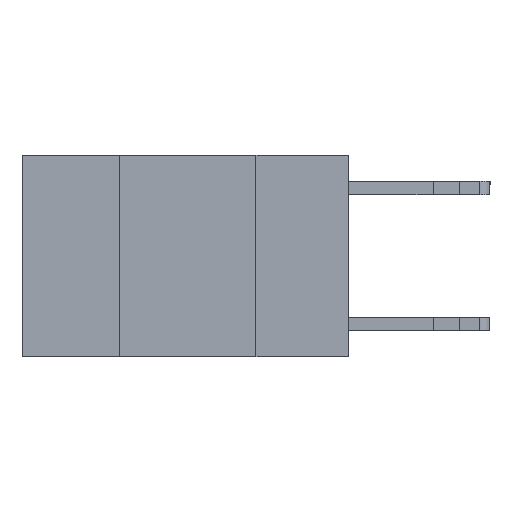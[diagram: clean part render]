
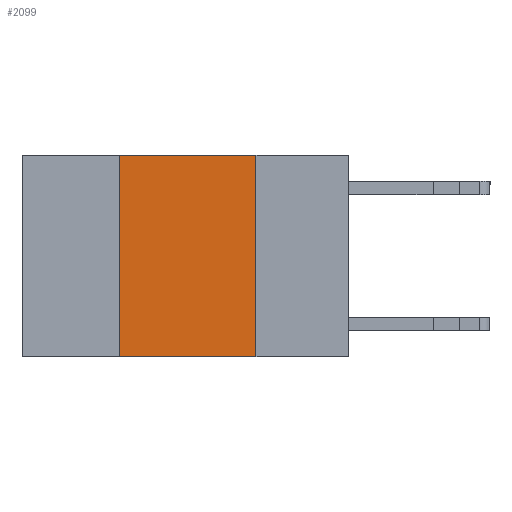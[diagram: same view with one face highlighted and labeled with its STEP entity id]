
A CAD part, left-side view. The second image highlights one B-rep face of the part: STEP entity #2099.
In plain terms, the highlighted planar face has unit normal (-1, 0, 0).
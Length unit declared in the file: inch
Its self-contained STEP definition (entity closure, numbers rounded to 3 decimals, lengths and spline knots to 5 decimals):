
#882 = CARTESIAN_POINT ( 'NONE',  ( 0., 0.17, -0.37 ) ) ;
#1571 = DIRECTION ( 'NONE',  ( 0., 0., -1. ) ) ;
#1668 = AXIS2_PLACEMENT_3D ( 'NONE', #8676, #10941, #1571 ) ;
#1819 = DIRECTION ( 'NONE',  ( 0., -1., 0. ) ) ;
#2099 = ADVANCED_FACE ( 'NONE', ( #13008 ), #7789, .F. ) ;
#2746 = ORIENTED_EDGE ( 'NONE', *, *, #3608, .F. ) ;
#3571 = VERTEX_POINT ( 'NONE', #882 ) ;
#3608 = EDGE_CURVE ( 'NONE', #10512, #7914, #11284, .T. ) ;
#3910 = CARTESIAN_POINT ( 'NONE',  ( 0., 0.17, 0. ) ) ;
#3930 = VECTOR ( 'NONE', #1819, 39.37008 ) ;
#4198 = EDGE_LOOP ( 'NONE', ( #11548, #12940, #2746, #7398 ) ) ;
#4563 = CARTESIAN_POINT ( 'NONE',  ( 0., 0.42, -0.37 ) ) ;
#4791 = VECTOR ( 'NONE', #10331, 39.37008 ) ;
#5809 = LINE ( 'NONE', #12005, #11822 ) ;
#6104 = EDGE_CURVE ( 'NONE', #7914, #10002, #5809, .T. ) ;
#6196 = EDGE_CURVE ( 'NONE', #10002, #3571, #8201, .T. ) ;
#7398 = ORIENTED_EDGE ( 'NONE', *, *, #12355, .T. ) ;
#7789 = PLANE ( 'NONE',  #1668 ) ;
#7914 = VERTEX_POINT ( 'NONE', #8962 ) ;
#8201 = LINE ( 'NONE', #3910, #4791 ) ;
#8676 = CARTESIAN_POINT ( 'NONE',  ( 0., 0.6, 0. ) ) ;
#8962 = CARTESIAN_POINT ( 'NONE',  ( 0., 0.42, 0. ) ) ;
#9032 = DIRECTION ( 'NONE',  ( 0., 0., 1. ) ) ;
#9234 = CARTESIAN_POINT ( 'NONE',  ( 0., 0.42, 0. ) ) ;
#9805 = DIRECTION ( 'NONE',  ( 0., -1., 0. ) ) ;
#10002 = VERTEX_POINT ( 'NONE', #12955 ) ;
#10331 = DIRECTION ( 'NONE',  ( 0., 0., -1. ) ) ;
#10512 = VERTEX_POINT ( 'NONE', #4563 ) ;
#10941 = DIRECTION ( 'NONE',  ( 1., 0., 0. ) ) ;
#11198 = CARTESIAN_POINT ( 'NONE',  ( 0., 0.6, -0.37 ) ) ;
#11284 = LINE ( 'NONE', #9234, #11762 ) ;
#11548 = ORIENTED_EDGE ( 'NONE', *, *, #6196, .F. ) ;
#11762 = VECTOR ( 'NONE', #9032, 39.37008 ) ;
#11822 = VECTOR ( 'NONE', #9805, 39.37008 ) ;
#12005 = CARTESIAN_POINT ( 'NONE',  ( 0., 0.6, 0. ) ) ;
#12355 = EDGE_CURVE ( 'NONE', #10512, #3571, #13251, .T. ) ;
#12940 = ORIENTED_EDGE ( 'NONE', *, *, #6104, .F. ) ;
#12955 = CARTESIAN_POINT ( 'NONE',  ( 0., 0.17, 0. ) ) ;
#13008 = FACE_OUTER_BOUND ( 'NONE', #4198, .T. ) ;
#13251 = LINE ( 'NONE', #11198, #3930 ) ;
